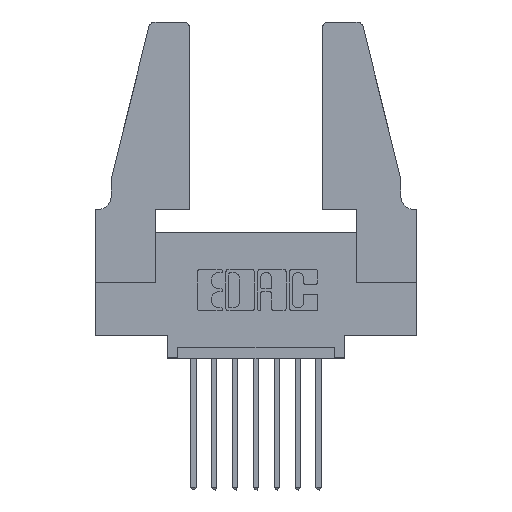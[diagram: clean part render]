
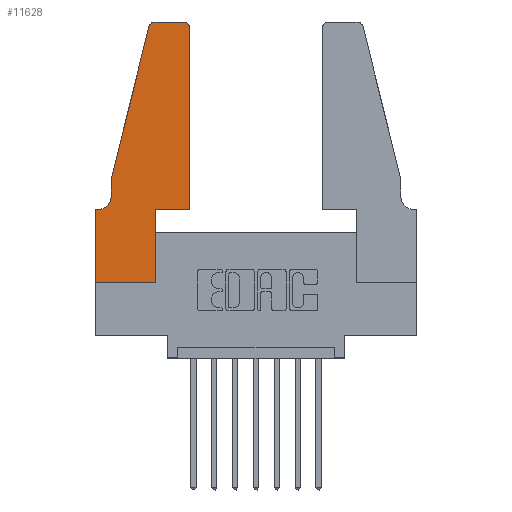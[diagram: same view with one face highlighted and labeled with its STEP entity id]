
A CAD part, top view. The second image highlights one B-rep face of the part: STEP entity #11628.
In plain terms, the highlighted planar face has unit normal (0, 0, 1).
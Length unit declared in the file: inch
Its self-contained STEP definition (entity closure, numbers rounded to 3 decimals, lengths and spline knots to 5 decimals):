
#21 = VERTEX_POINT ( 'NONE', #9804 ) ;
#156 = DIRECTION ( 'NONE',  ( 0., -1., 0. ) ) ;
#229 = EDGE_CURVE ( 'NONE', #804, #5665, #1467, .T. ) ;
#295 = LINE ( 'NONE', #9581, #12032 ) ;
#320 = VERTEX_POINT ( 'NONE', #1964 ) ;
#382 = DIRECTION ( 'NONE',  ( 1., 0., 0. ) ) ;
#400 = EDGE_CURVE ( 'NONE', #320, #11464, #9911, .T. ) ;
#470 = ORIENTED_EDGE ( 'NONE', *, *, #400, .T. ) ;
#586 = DIRECTION ( 'NONE',  ( -1., 0., 0. ) ) ;
#804 = VERTEX_POINT ( 'NONE', #4424 ) ;
#823 = DIRECTION ( 'NONE',  ( -1., 0., 0. ) ) ;
#836 = VECTOR ( 'NONE', #7902, 39.37008 ) ;
#842 = DIRECTION ( 'NONE',  ( 0., 0., 1. ) ) ;
#878 = VECTOR ( 'NONE', #1888, 39.37008 ) ;
#937 = VERTEX_POINT ( 'NONE', #8384 ) ;
#1171 = CARTESIAN_POINT ( 'NONE',  ( 0.0755, 0.35, 0.37 ) ) ;
#1363 = VERTEX_POINT ( 'NONE', #11088 ) ;
#1439 = CARTESIAN_POINT ( 'NONE',  ( 0., 0., 0.37 ) ) ;
#1467 = CIRCLE ( 'NONE', #6533, 0.07 ) ;
#1693 = DIRECTION ( 'NONE',  ( 0., 0., -1. ) ) ;
#1707 = CARTESIAN_POINT ( 'NONE',  ( 0.4205, 1.25, 0.37 ) ) ;
#1774 = EDGE_CURVE ( 'NONE', #12191, #9652, #7621, .T. ) ;
#1798 = EDGE_CURVE ( 'NONE', #2514, #7061, #8249, .T. ) ;
#1888 = DIRECTION ( 'NONE',  ( 0., 1., 0. ) ) ;
#1909 = PLANE ( 'NONE',  #8805 ) ;
#1935 = CARTESIAN_POINT ( 'NONE',  ( 0., 0.35, 0.37 ) ) ;
#1964 = CARTESIAN_POINT ( 'NONE',  ( 0.2865, 0., 0.37 ) ) ;
#2077 = ORIENTED_EDGE ( 'NONE', *, *, #4700, .T. ) ;
#2155 = VECTOR ( 'NONE', #586, 39.37008 ) ;
#2377 = ORIENTED_EDGE ( 'NONE', *, *, #10291, .T. ) ;
#2434 = CARTESIAN_POINT ( 'NONE',  ( 0.4505, 1.22, 0.37 ) ) ;
#2514 = VERTEX_POINT ( 'NONE', #11269 ) ;
#3035 = LINE ( 'NONE', #1171, #836 ) ;
#3072 = LINE ( 'NONE', #1439, #6164 ) ;
#3349 = VERTEX_POINT ( 'NONE', #1935 ) ;
#3383 = AXIS2_PLACEMENT_3D ( 'NONE', #4632, #842, #12200 ) ;
#3685 = CARTESIAN_POINT ( 'NONE',  ( 0.0755, 0.5, 0.37 ) ) ;
#3721 = ORIENTED_EDGE ( 'NONE', *, *, #8616, .T. ) ;
#3736 = CIRCLE ( 'NONE', #3383, 0.03 ) ;
#3890 = DIRECTION ( 'NONE',  ( 1., 0., 0. ) ) ;
#4378 = VECTOR ( 'NONE', #156, 39.37008 ) ;
#4424 = CARTESIAN_POINT ( 'NONE',  ( 0.0755, 0.42, 0.37 ) ) ;
#4507 = CARTESIAN_POINT ( 'NONE',  ( 0.0755, 0.5, 0.37 ) ) ;
#4632 = CARTESIAN_POINT ( 'NONE',  ( 0.4205, 1.22, 0.37 ) ) ;
#4700 = EDGE_CURVE ( 'NONE', #937, #804, #7112, .T. ) ;
#5107 = DIRECTION ( 'NONE',  ( 0., 0., 1. ) ) ;
#5123 = ORIENTED_EDGE ( 'NONE', *, *, #1798, .T. ) ;
#5205 = VECTOR ( 'NONE', #8197, 39.37008 ) ;
#5286 = DIRECTION ( 'NONE',  ( 1., 0., 0. ) ) ;
#5370 = ORIENTED_EDGE ( 'NONE', *, *, #7955, .T. ) ;
#5665 = VERTEX_POINT ( 'NONE', #6934 ) ;
#5832 = VECTOR ( 'NONE', #8299, 39.37008 ) ;
#6164 = VECTOR ( 'NONE', #7921, 39.37008 ) ;
#6315 = AXIS2_PLACEMENT_3D ( 'NONE', #7945, #5107, #382 ) ;
#6533 = AXIS2_PLACEMENT_3D ( 'NONE', #11179, #1693, #823 ) ;
#6595 = EDGE_CURVE ( 'NONE', #1363, #320, #3072, .T. ) ;
#6735 = CARTESIAN_POINT ( 'NONE',  ( 0., 0., 0.37 ) ) ;
#6934 = CARTESIAN_POINT ( 'NONE',  ( 0.0055, 0.35, 0.37 ) ) ;
#6993 = CARTESIAN_POINT ( 'NONE',  ( 0.284, 1.25, 0.37 ) ) ;
#7061 = VERTEX_POINT ( 'NONE', #2434 ) ;
#7112 = LINE ( 'NONE', #4507, #5205 ) ;
#7155 = CARTESIAN_POINT ( 'NONE',  ( 0.2605, 1.25, 0.37 ) ) ;
#7427 = VECTOR ( 'NONE', #12167, 39.37008 ) ;
#7621 = LINE ( 'NONE', #7155, #2155 ) ;
#7813 = ORIENTED_EDGE ( 'NONE', *, *, #1774, .T. ) ;
#7902 = DIRECTION ( 'NONE',  ( -1., 0., 0. ) ) ;
#7921 = DIRECTION ( 'NONE',  ( 1., 0., 0. ) ) ;
#7945 = CARTESIAN_POINT ( 'NONE',  ( 0.284, 1.22, 0.37 ) ) ;
#7955 = EDGE_CURVE ( 'NONE', #3349, #1363, #11362, .T. ) ;
#8099 = DIRECTION ( 'NONE',  ( 0., 0., 1. ) ) ;
#8117 = CARTESIAN_POINT ( 'NONE',  ( 0.4505, 0.35, 0.37 ) ) ;
#8197 = DIRECTION ( 'NONE',  ( 0., -1., 0. ) ) ;
#8249 = LINE ( 'NONE', #8117, #5832 ) ;
#8299 = DIRECTION ( 'NONE',  ( 0., 1., 0. ) ) ;
#8384 = CARTESIAN_POINT ( 'NONE',  ( 0.0755, 0.5, 0.37 ) ) ;
#8424 = EDGE_CURVE ( 'NONE', #5665, #3349, #3035, .T. ) ;
#8547 = ORIENTED_EDGE ( 'NONE', *, *, #229, .T. ) ;
#8616 = EDGE_CURVE ( 'NONE', #7061, #12191, #3736, .T. ) ;
#8630 = ORIENTED_EDGE ( 'NONE', *, *, #6595, .T. ) ;
#8805 = AXIS2_PLACEMENT_3D ( 'NONE', #10811, #8099, #5286 ) ;
#9057 = FACE_OUTER_BOUND ( 'NONE', #10028, .T. ) ;
#9252 = ORIENTED_EDGE ( 'NONE', *, *, #10995, .T. ) ;
#9367 = LINE ( 'NONE', #3685, #7427 ) ;
#9581 = CARTESIAN_POINT ( 'NONE',  ( 0.4505, 0.35, 0.37 ) ) ;
#9652 = VERTEX_POINT ( 'NONE', #6993 ) ;
#9804 = CARTESIAN_POINT ( 'NONE',  ( 0.25487, 1.22718, 0.37 ) ) ;
#9911 = LINE ( 'NONE', #11300, #878 ) ;
#10028 = EDGE_LOOP ( 'NONE', ( #7813, #11141, #2377, #2077, #8547, #10243, #5370, #8630, #470, #9252, #5123, #3721 ) ) ;
#10243 = ORIENTED_EDGE ( 'NONE', *, *, #8424, .T. ) ;
#10291 = EDGE_CURVE ( 'NONE', #21, #937, #9367, .T. ) ;
#10811 = CARTESIAN_POINT ( 'NONE',  ( 0., 0.35, 0.37 ) ) ;
#10995 = EDGE_CURVE ( 'NONE', #11464, #2514, #295, .T. ) ;
#11020 = EDGE_CURVE ( 'NONE', #9652, #21, #12196, .T. ) ;
#11088 = CARTESIAN_POINT ( 'NONE',  ( 0., 0., 0.37 ) ) ;
#11141 = ORIENTED_EDGE ( 'NONE', *, *, #11020, .T. ) ;
#11179 = CARTESIAN_POINT ( 'NONE',  ( 0.0055, 0.42, 0.37 ) ) ;
#11269 = CARTESIAN_POINT ( 'NONE',  ( 0.4505, 0.35, 0.37 ) ) ;
#11300 = CARTESIAN_POINT ( 'NONE',  ( 0.2865, 0.35, 0.37 ) ) ;
#11362 = LINE ( 'NONE', #6735, #4378 ) ;
#11464 = VERTEX_POINT ( 'NONE', #11550 ) ;
#11550 = CARTESIAN_POINT ( 'NONE',  ( 0.2865, 0.35, 0.37 ) ) ;
#11628 = ADVANCED_FACE ( 'NONE', ( #9057 ), #1909, .T. ) ;
#12032 = VECTOR ( 'NONE', #3890, 39.37008 ) ;
#12167 = DIRECTION ( 'NONE',  ( -0.239, -0.971, 0. ) ) ;
#12191 = VERTEX_POINT ( 'NONE', #1707 ) ;
#12196 = CIRCLE ( 'NONE', #6315, 0.03 ) ;
#12200 = DIRECTION ( 'NONE',  ( 1., 0., 0. ) ) ;
